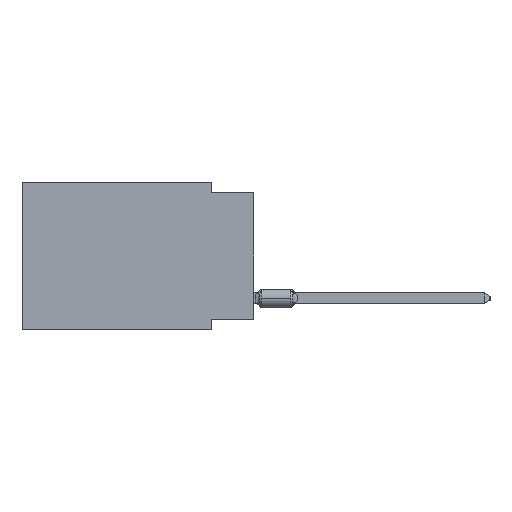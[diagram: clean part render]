
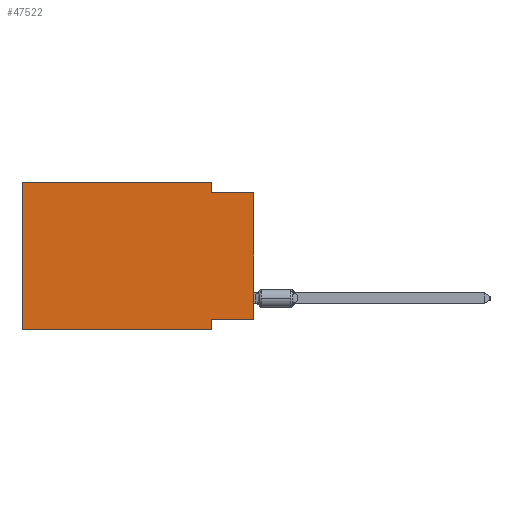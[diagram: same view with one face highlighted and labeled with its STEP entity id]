
A CAD part, left-side view. The second image highlights one B-rep face of the part: STEP entity #47522.
In plain terms, the highlighted planar face has unit normal (-1, 0, 0).
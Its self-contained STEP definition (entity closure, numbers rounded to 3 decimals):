
#819 = EDGE_CURVE ( 'NONE', #11317, #13734, #8150, .T. ) ;
#1699 = VERTEX_POINT ( 'NONE', #8606 ) ;
#5804 = ORIENTED_EDGE ( 'NONE', *, *, #56962, .T. ) ;
#7624 = ORIENTED_EDGE ( 'NONE', *, *, #27379, .F. ) ;
#7961 = VERTEX_POINT ( 'NONE', #31691 ) ;
#8150 = LINE ( 'NONE', #36506, #23614 ) ;
#8606 = CARTESIAN_POINT ( 'NONE',  ( 0., 2.54, 0. ) ) ;
#10342 = CARTESIAN_POINT ( 'NONE',  ( 0., 0., -0.635 ) ) ;
#11317 = VERTEX_POINT ( 'NONE', #32674 ) ;
#11609 = VECTOR ( 'NONE', #62982, 1000. ) ;
#12040 = CARTESIAN_POINT ( 'NONE',  ( 0., 0., -8.255 ) ) ;
#12683 = DIRECTION ( 'NONE',  ( 0., 0., -1. ) ) ;
#13734 = VERTEX_POINT ( 'NONE', #29438 ) ;
#18347 = LINE ( 'NONE', #41481, #69057 ) ;
#20745 = EDGE_CURVE ( 'NONE', #7961, #1699, #24687, .T. ) ;
#22463 = LINE ( 'NONE', #38530, #73145 ) ;
#23614 = VECTOR ( 'NONE', #42841, 1000. ) ;
#24687 = LINE ( 'NONE', #64996, #38485 ) ;
#25523 = CARTESIAN_POINT ( 'NONE',  ( 0., 2.54, -0.635 ) ) ;
#25861 = AXIS2_PLACEMENT_3D ( 'NONE', #63838, #69426, #12683 ) ;
#27379 = EDGE_CURVE ( 'NONE', #58499, #55016, #33126, .T. ) ;
#29390 = LINE ( 'NONE', #46553, #68073 ) ;
#29438 = CARTESIAN_POINT ( 'NONE',  ( 0., 2.54, -8.89 ) ) ;
#30184 = ORIENTED_EDGE ( 'NONE', *, *, #819, .F. ) ;
#30476 = VECTOR ( 'NONE', #61953, 1000. ) ;
#31005 = CARTESIAN_POINT ( 'NONE',  ( 0., 0., -8.255 ) ) ;
#31691 = CARTESIAN_POINT ( 'NONE',  ( 0., 13.97, 0. ) ) ;
#32674 = CARTESIAN_POINT ( 'NONE',  ( 0., 2.54, -8.255 ) ) ;
#33126 = LINE ( 'NONE', #44697, #11609 ) ;
#33708 = EDGE_LOOP ( 'NONE', ( #5804, #7624, #38197, #66864, #70327, #49586, #30184, #70047 ) ) ;
#35809 = FACE_OUTER_BOUND ( 'NONE', #33708, .T. ) ;
#36021 = CARTESIAN_POINT ( 'NONE',  ( 0., 13.97, -8.89 ) ) ;
#36506 = CARTESIAN_POINT ( 'NONE',  ( 0., 2.54, -8.89 ) ) ;
#37346 = DIRECTION ( 'NONE',  ( 0., -1., 0. ) ) ;
#38197 = ORIENTED_EDGE ( 'NONE', *, *, #73905, .F. ) ;
#38485 = VECTOR ( 'NONE', #37346, 1000. ) ;
#38530 = CARTESIAN_POINT ( 'NONE',  ( 0., 0., 0. ) ) ;
#40394 = LINE ( 'NONE', #12040, #42830 ) ;
#41034 = PLANE ( 'NONE',  #25861 ) ;
#41203 = EDGE_CURVE ( 'NONE', #72951, #11317, #40394, .T. ) ;
#41481 = CARTESIAN_POINT ( 'NONE',  ( 0., 2.54, 0. ) ) ;
#42830 = VECTOR ( 'NONE', #53098, 1000. ) ;
#42841 = DIRECTION ( 'NONE',  ( 0., 0., -1. ) ) ;
#44065 = VERTEX_POINT ( 'NONE', #36021 ) ;
#44397 = LINE ( 'NONE', #50363, #30476 ) ;
#44697 = CARTESIAN_POINT ( 'NONE',  ( 0., 0., -0.635 ) ) ;
#46553 = CARTESIAN_POINT ( 'NONE',  ( 0., 13.97, -8.89 ) ) ;
#47522 = ADVANCED_FACE ( 'NONE', ( #35809 ), #41034, .F. ) ;
#49586 = ORIENTED_EDGE ( 'NONE', *, *, #50576, .T. ) ;
#50363 = CARTESIAN_POINT ( 'NONE',  ( 0., 13.97, 0. ) ) ;
#50459 = DIRECTION ( 'NONE',  ( 0., 0., 1. ) ) ;
#50576 = EDGE_CURVE ( 'NONE', #44065, #13734, #29390, .T. ) ;
#52157 = DIRECTION ( 'NONE',  ( 0., -1., 0. ) ) ;
#53098 = DIRECTION ( 'NONE',  ( 0., 1., 0. ) ) ;
#55016 = VERTEX_POINT ( 'NONE', #10342 ) ;
#56962 = EDGE_CURVE ( 'NONE', #72951, #55016, #22463, .T. ) ;
#58499 = VERTEX_POINT ( 'NONE', #25523 ) ;
#61953 = DIRECTION ( 'NONE',  ( 0., 0., 1. ) ) ;
#62982 = DIRECTION ( 'NONE',  ( 0., -1., 0. ) ) ;
#63838 = CARTESIAN_POINT ( 'NONE',  ( 0., 13.97, 0. ) ) ;
#63901 = DIRECTION ( 'NONE',  ( 0., 0., -1. ) ) ;
#64996 = CARTESIAN_POINT ( 'NONE',  ( 0., 13.97, 0. ) ) ;
#66864 = ORIENTED_EDGE ( 'NONE', *, *, #20745, .F. ) ;
#68073 = VECTOR ( 'NONE', #52157, 1000. ) ;
#68128 = EDGE_CURVE ( 'NONE', #44065, #7961, #44397, .T. ) ;
#69057 = VECTOR ( 'NONE', #63901, 1000. ) ;
#69426 = DIRECTION ( 'NONE',  ( 1., 0., 0. ) ) ;
#70047 = ORIENTED_EDGE ( 'NONE', *, *, #41203, .F. ) ;
#70327 = ORIENTED_EDGE ( 'NONE', *, *, #68128, .F. ) ;
#72951 = VERTEX_POINT ( 'NONE', #31005 ) ;
#73145 = VECTOR ( 'NONE', #50459, 1000. ) ;
#73905 = EDGE_CURVE ( 'NONE', #1699, #58499, #18347, .T. ) ;
